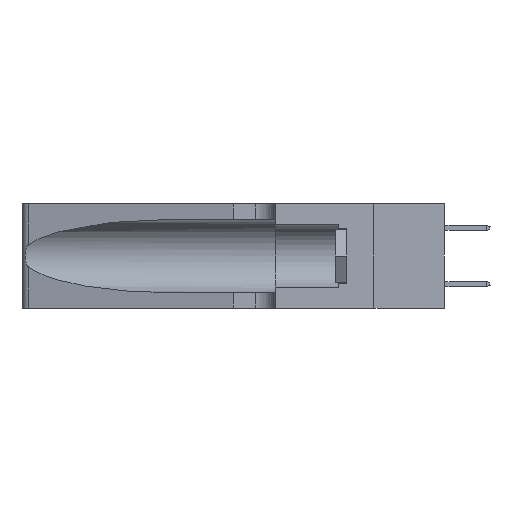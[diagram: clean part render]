
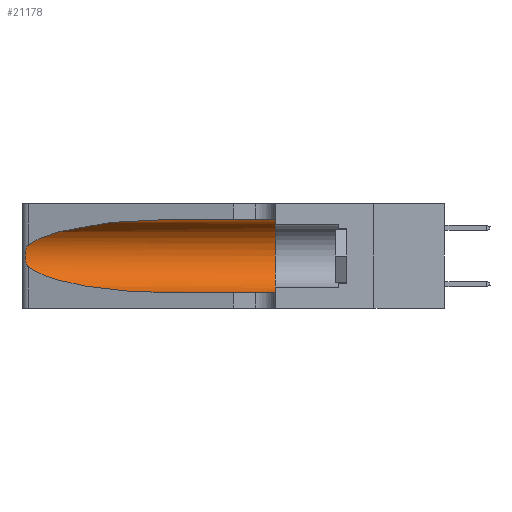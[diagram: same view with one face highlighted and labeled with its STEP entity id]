
A CAD part, left-side view. The second image highlights one B-rep face of the part: STEP entity #21178.
In plain terms, the highlighted cylindrical face has radius 3.308 mm (diameter 6.617 mm), a partial arc.
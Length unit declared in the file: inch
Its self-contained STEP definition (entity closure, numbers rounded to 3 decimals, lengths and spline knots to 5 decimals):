
#49 = CARTESIAN_POINT ( 'NONE',  ( 0.26018, 1.23835, 0.19895 ) ) ;
#63 = VERTEX_POINT ( 'NONE', #20870 ) ;
#397 = CARTESIAN_POINT ( 'NONE',  ( 0.25487, 1.22718, 0.14631 ) ) ;
#846 = CARTESIAN_POINT ( 'NONE',  ( 0.25487, 1.22718, 0.14631 ) ) ;
#1885 = EDGE_CURVE ( 'NONE', #29134, #4891, #15760, .T. ) ;
#2749 = ORIENTED_EDGE ( 'NONE', *, *, #22018, .T. ) ;
#3282 = CYLINDRICAL_SURFACE ( 'NONE', #27025, 0.13025 ) ;
#4755 = LINE ( 'NONE', #25620, #32468 ) ;
#4891 = VERTEX_POINT ( 'NONE', #7845 ) ;
#5361 = ORIENTED_EDGE ( 'NONE', *, *, #15645, .F. ) ;
#6484 = CARTESIAN_POINT ( 'NONE',  ( 0.25856, 1.23593, 0.16098 ) ) ;
#7845 = CARTESIAN_POINT ( 'NONE',  ( 0.25487, 1.22718, 0.14631 ) ) ;
#8736 = CARTESIAN_POINT ( 'NONE',  ( 0.26075, 1.23896, 0.178 ) ) ;
#10065 = CARTESIAN_POINT ( 'NONE',  ( 0.18966, 0.96281, 0.05475 ) ) ;
#10963 = DIRECTION ( 'NONE',  ( 0., -1., 0. ) ) ;
#12363 = CARTESIAN_POINT ( 'NONE',  ( 0.25639, 1.23186, 0.15144 ) ) ;
#13070 = ORIENTED_EDGE ( 'NONE', *, *, #34143, .T. ) ;
#13399 = ORIENTED_EDGE ( 'NONE', *, *, #36476, .T. ) ;
#13778 = CIRCLE ( 'NONE', #36978, 0.13025 ) ;
#15645 = EDGE_CURVE ( 'NONE', #20261, #63, #26393, .T. ) ;
#15712 = CARTESIAN_POINT ( 'NONE',  ( 0.25487, 1.22718, 0.22369 ) ) ;
#15760 = B_SPLINE_CURVE_WITH_KNOTS ( 'NONE', 3,
 ( #36449, #36824, #34528, #17159, #34172, #49, #22955, #8736, #32138, #6484, #26565, #12363, #34776, #397 ),
 .UNSPECIFIED., .F., .F.,
 ( 4, 2, 2, 2, 2, 2, 4 ),
 ( 0., 0.00027, 0.00053, 0.00107, 0.0016, 0.00187, 0.00214 ),
 .UNSPECIFIED. ) ;
#16013 = VERTEX_POINT ( 'NONE', #22423 ) ;
#16114 = DIRECTION ( 'NONE',  ( 0., 1., 0. ) ) ;
#16492 = VECTOR ( 'NONE', #10963, 39.37008 ) ;
#17159 = CARTESIAN_POINT ( 'NONE',  ( 0.25787, 1.23484, 0.2124 ) ) ;
#18103 = CARTESIAN_POINT ( 'NONE',  ( 0.1305, 0.72297, 0.05475 ) ) ;
#19240 = DIRECTION ( 'NONE',  ( 0., 0., 1. ) ) ;
#19463 = CARTESIAN_POINT ( 'NONE',  ( 0.25487, 1.22718, 0.22369 ) ) ;
#19961 = DIRECTION ( 'NONE',  ( 0., -1., 0. ) ) ;
#20261 = VERTEX_POINT ( 'NONE', #25315 ) ;
#20870 = CARTESIAN_POINT ( 'NONE',  ( 0.1305, 0.35, 0.31525 ) ) ;
#20933 = VERTEX_POINT ( 'NONE', #27541 ) ;
#21178 = ADVANCED_FACE ( 'NONE', ( #26680 ), #3282, .F. ) ;
#22018 = EDGE_CURVE ( 'NONE', #4891, #16013, #24040, .T. ) ;
#22423 = CARTESIAN_POINT ( 'NONE',  ( 0.1305, 0.72297, 0.05475 ) ) ;
#22955 = CARTESIAN_POINT ( 'NONE',  ( 0.26075, 1.23896, 0.19203 ) ) ;
#24040 =( BOUNDED_CURVE ( )  B_SPLINE_CURVE ( 3, ( #846, #32339, #10065, #18103 ),
 .UNSPECIFIED., .F., .F. ) 
 B_SPLINE_CURVE_WITH_KNOTS ( ( 4, 4 ),
 ( 3.44316, 4.71239 ),
 .UNSPECIFIED. ) 
 CURVE ( )  GEOMETRIC_REPRESENTATION_ITEM ( )  RATIONAL_B_SPLINE_CURVE ( ( 1., 0.87, 0.87, 1. ) ) 
 REPRESENTATION_ITEM ( '' )  );
#25214 =( BOUNDED_CURVE ( )  B_SPLINE_CURVE ( 3, ( #27128, #32690, #35729, #15712 ),
 .UNSPECIFIED., .F., .F. ) 
 B_SPLINE_CURVE_WITH_KNOTS ( ( 4, 4 ),
 ( 1.5708, 2.84003 ),
 .UNSPECIFIED. ) 
 CURVE ( )  GEOMETRIC_REPRESENTATION_ITEM ( )  RATIONAL_B_SPLINE_CURVE ( ( 1., 0.87, 0.87, 1. ) ) 
 REPRESENTATION_ITEM ( '' )  );
#25315 = CARTESIAN_POINT ( 'NONE',  ( 0.1305, 0.72297, 0.31525 ) ) ;
#25620 = CARTESIAN_POINT ( 'NONE',  ( 0.1305, 1.61858, 0.05475 ) ) ;
#25942 = ORIENTED_EDGE ( 'NONE', *, *, #1885, .T. ) ;
#26393 = LINE ( 'NONE', #26678, #16492 ) ;
#26401 = DIRECTION ( 'NONE',  ( 0., -1., 0. ) ) ;
#26565 = CARTESIAN_POINT ( 'NONE',  ( 0.25789, 1.23486, 0.15765 ) ) ;
#26678 = CARTESIAN_POINT ( 'NONE',  ( 0.1305, 1.61858, 0.31525 ) ) ;
#26680 = FACE_OUTER_BOUND ( 'NONE', #33333, .T. ) ;
#27025 = AXIS2_PLACEMENT_3D ( 'NONE', #34742, #26401, #32105 ) ;
#27128 = CARTESIAN_POINT ( 'NONE',  ( 0.1305, 0.72297, 0.31525 ) ) ;
#27541 = CARTESIAN_POINT ( 'NONE',  ( 0.1305, 0.35, 0.05475 ) ) ;
#28675 = EDGE_CURVE ( 'NONE', #63, #20933, #13778, .T. ) ;
#29134 = VERTEX_POINT ( 'NONE', #19463 ) ;
#32105 = DIRECTION ( 'NONE',  ( 0., 0., -1. ) ) ;
#32138 = CARTESIAN_POINT ( 'NONE',  ( 0.26017, 1.23833, 0.17102 ) ) ;
#32339 = CARTESIAN_POINT ( 'NONE',  ( 0.2373, 1.15595, 0.08982 ) ) ;
#32468 = VECTOR ( 'NONE', #19961, 39.37008 ) ;
#32482 = ORIENTED_EDGE ( 'NONE', *, *, #28675, .F. ) ;
#32690 = CARTESIAN_POINT ( 'NONE',  ( 0.18966, 0.96281, 0.31525 ) ) ;
#33333 = EDGE_LOOP ( 'NONE', ( #13070, #25942, #2749, #13399, #32482, #5361 ) ) ;
#33586 = CARTESIAN_POINT ( 'NONE',  ( 0.1305, 0.35, 0.185 ) ) ;
#34143 = EDGE_CURVE ( 'NONE', #20261, #29134, #25214, .T. ) ;
#34172 = CARTESIAN_POINT ( 'NONE',  ( 0.25854, 1.2359, 0.20912 ) ) ;
#34528 = CARTESIAN_POINT ( 'NONE',  ( 0.25639, 1.23184, 0.21858 ) ) ;
#34742 = CARTESIAN_POINT ( 'NONE',  ( 0.1305, 1.61858, 0.185 ) ) ;
#34776 = CARTESIAN_POINT ( 'NONE',  ( 0.25555, 1.22993, 0.14849 ) ) ;
#35729 = CARTESIAN_POINT ( 'NONE',  ( 0.2373, 1.15595, 0.28018 ) ) ;
#36449 = CARTESIAN_POINT ( 'NONE',  ( 0.25487, 1.22718, 0.22369 ) ) ;
#36476 = EDGE_CURVE ( 'NONE', #16013, #20933, #4755, .T. ) ;
#36824 = CARTESIAN_POINT ( 'NONE',  ( 0.25555, 1.22994, 0.2215 ) ) ;
#36978 = AXIS2_PLACEMENT_3D ( 'NONE', #33586, #16114, #19240 ) ;
